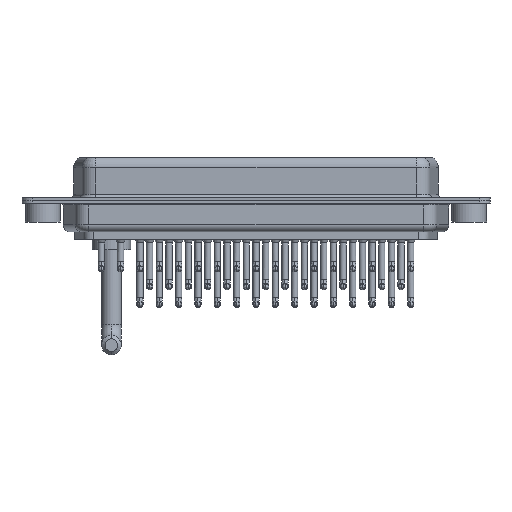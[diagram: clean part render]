
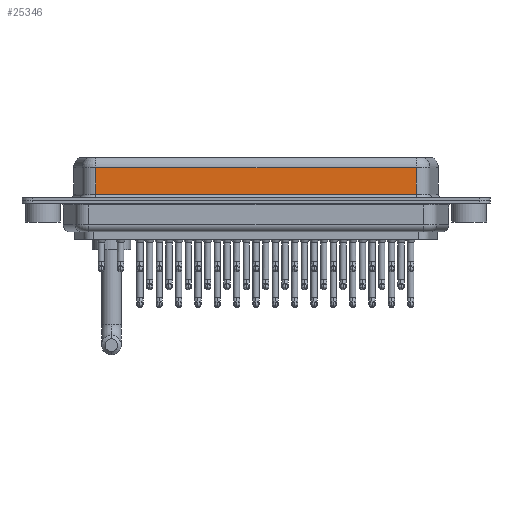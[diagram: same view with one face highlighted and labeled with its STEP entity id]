
A CAD part, front view. The second image highlights one B-rep face of the part: STEP entity #25346.
In plain terms, the highlighted planar face has unit normal (0, -1, 0).
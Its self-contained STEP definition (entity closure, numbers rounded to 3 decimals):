
#140 = CARTESIAN_POINT ( 'NONE',  ( 53.41, -5.375, 4.65 ) ) ;
#2304 = LINE ( 'NONE', #20333, #30783 ) ;
#2856 = CARTESIAN_POINT ( 'NONE',  ( 53.41, -5.375, 6.4 ) ) ;
#5154 = AXIS2_PLACEMENT_3D ( 'NONE', #2856, #10418, #31859 ) ;
#5439 = PLANE ( 'NONE',  #5154 ) ;
#5443 = LINE ( 'NONE', #16603, #9239 ) ;
#5837 = VERTEX_POINT ( 'NONE', #22013 ) ;
#5999 = CARTESIAN_POINT ( 'NONE',  ( 7.59, -5.375, 6.4 ) ) ;
#6450 = CARTESIAN_POINT ( 'NONE',  ( 7.59, -5.375, 4.65 ) ) ;
#6553 = EDGE_CURVE ( 'NONE', #9310, #8663, #23490, .T. ) ;
#7668 = FACE_OUTER_BOUND ( 'NONE', #28081, .T. ) ;
#8663 = VERTEX_POINT ( 'NONE', #6450 ) ;
#9239 = VECTOR ( 'NONE', #15920, 1000. ) ;
#9310 = VERTEX_POINT ( 'NONE', #20431 ) ;
#10418 = DIRECTION ( 'NONE',  ( 0., 1., 0. ) ) ;
#10805 = DIRECTION ( 'NONE',  ( 0., 0., -1. ) ) ;
#10974 = LINE ( 'NONE', #5999, #29882 ) ;
#13530 = DIRECTION ( 'NONE',  ( -1., 0., 0. ) ) ;
#14945 = VECTOR ( 'NONE', #13530, 1000. ) ;
#15920 = DIRECTION ( 'NONE',  ( 1., 0., 0. ) ) ;
#16603 = CARTESIAN_POINT ( 'NONE',  ( 53.41, -5.375, 0.9 ) ) ;
#19265 = EDGE_CURVE ( 'NONE', #9310, #5837, #2304, .T. ) ;
#20333 = CARTESIAN_POINT ( 'NONE',  ( 53.41, -5.375, 6.4 ) ) ;
#20431 = CARTESIAN_POINT ( 'NONE',  ( 53.41, -5.375, 4.65 ) ) ;
#22013 = CARTESIAN_POINT ( 'NONE',  ( 53.41, -5.375, 0.9 ) ) ;
#22539 = EDGE_CURVE ( 'NONE', #8663, #26004, #10974, .T. ) ;
#22732 = DIRECTION ( 'NONE',  ( 0., 0., -1. ) ) ;
#22799 = ORIENTED_EDGE ( 'NONE', *, *, #19265, .F. ) ;
#23490 = LINE ( 'NONE', #140, #14945 ) ;
#25346 = ADVANCED_FACE ( 'NONE', ( #7668 ), #5439, .F. ) ;
#26004 = VERTEX_POINT ( 'NONE', #28489 ) ;
#26959 = ORIENTED_EDGE ( 'NONE', *, *, #6553, .T. ) ;
#28081 = EDGE_LOOP ( 'NONE', ( #22799, #26959, #30951, #32365 ) ) ;
#28489 = CARTESIAN_POINT ( 'NONE',  ( 7.59, -5.375, 0.9 ) ) ;
#29882 = VECTOR ( 'NONE', #10805, 1000. ) ;
#30690 = EDGE_CURVE ( 'NONE', #26004, #5837, #5443, .T. ) ;
#30783 = VECTOR ( 'NONE', #22732, 1000. ) ;
#30951 = ORIENTED_EDGE ( 'NONE', *, *, #22539, .T. ) ;
#31859 = DIRECTION ( 'NONE',  ( 0., 0., 1. ) ) ;
#32365 = ORIENTED_EDGE ( 'NONE', *, *, #30690, .T. ) ;
